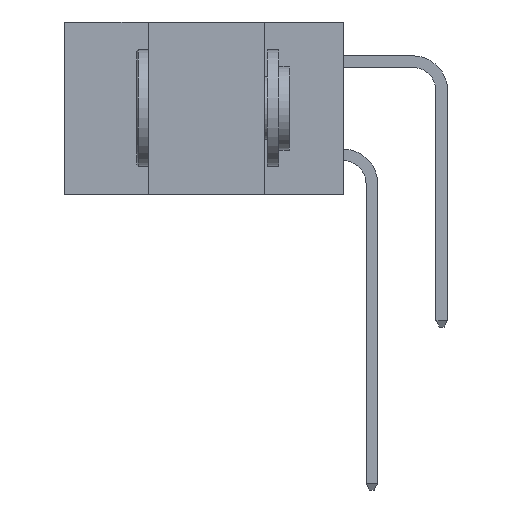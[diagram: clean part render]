
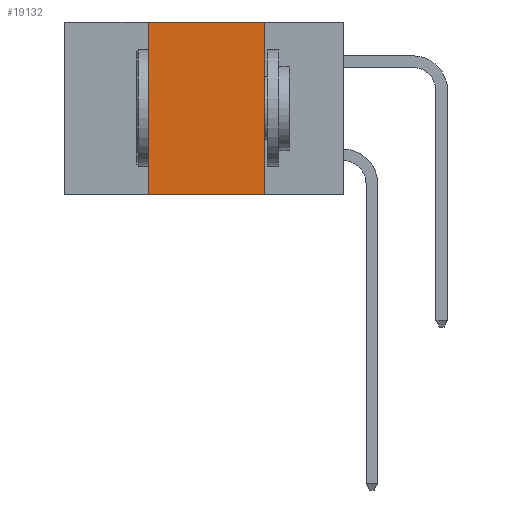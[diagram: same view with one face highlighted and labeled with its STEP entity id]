
A CAD part, left-side view. The second image highlights one B-rep face of the part: STEP entity #19132.
In plain terms, the highlighted planar face has unit normal (-1, 0, 0).
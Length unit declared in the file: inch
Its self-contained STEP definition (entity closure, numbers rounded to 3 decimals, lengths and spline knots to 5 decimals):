
#700 = CARTESIAN_POINT ( 'NONE',  ( 0., 0.6, 0. ) ) ;
#1573 = LINE ( 'NONE', #16615, #20217 ) ;
#2602 = DIRECTION ( 'NONE',  ( 1., 0., 0. ) ) ;
#3029 = ORIENTED_EDGE ( 'NONE', *, *, #15381, .T. ) ;
#3266 = VERTEX_POINT ( 'NONE', #19414 ) ;
#3692 = DIRECTION ( 'NONE',  ( 0., -1., 0. ) ) ;
#5593 = ORIENTED_EDGE ( 'NONE', *, *, #17843, .F. ) ;
#5947 = DIRECTION ( 'NONE',  ( 0., 0., -1. ) ) ;
#6161 = ORIENTED_EDGE ( 'NONE', *, *, #16584, .F. ) ;
#6325 = CARTESIAN_POINT ( 'NONE',  ( 0., 0.6, -0.37 ) ) ;
#7026 = FACE_OUTER_BOUND ( 'NONE', #20776, .T. ) ;
#7768 = DIRECTION ( 'NONE',  ( 0., 0., 1. ) ) ;
#7866 = VERTEX_POINT ( 'NONE', #9496 ) ;
#8141 = DIRECTION ( 'NONE',  ( 0., -1., 0. ) ) ;
#8465 = LINE ( 'NONE', #6325, #17462 ) ;
#8709 = VECTOR ( 'NONE', #5947, 39.37008 ) ;
#9181 = VECTOR ( 'NONE', #3692, 39.37008 ) ;
#9196 = VERTEX_POINT ( 'NONE', #13192 ) ;
#9496 = CARTESIAN_POINT ( 'NONE',  ( 0., 0.42, -0.37 ) ) ;
#10321 = AXIS2_PLACEMENT_3D ( 'NONE', #700, #2602, #15175 ) ;
#11581 = PLANE ( 'NONE',  #10321 ) ;
#13192 = CARTESIAN_POINT ( 'NONE',  ( 0., 0.17, 0. ) ) ;
#13944 = LINE ( 'NONE', #21557, #9181 ) ;
#15175 = DIRECTION ( 'NONE',  ( 0., 0., -1. ) ) ;
#15381 = EDGE_CURVE ( 'NONE', #7866, #3266, #8465, .T. ) ;
#16584 = EDGE_CURVE ( 'NONE', #7866, #19836, #1573, .T. ) ;
#16615 = CARTESIAN_POINT ( 'NONE',  ( 0., 0.42, -0.37 ) ) ;
#16671 = CARTESIAN_POINT ( 'NONE',  ( 0., 0.17, -0.37 ) ) ;
#16973 = CARTESIAN_POINT ( 'NONE',  ( 0., 0.42, 0. ) ) ;
#17462 = VECTOR ( 'NONE', #8141, 39.37008 ) ;
#17843 = EDGE_CURVE ( 'NONE', #19836, #9196, #13944, .T. ) ;
#19027 = EDGE_CURVE ( 'NONE', #9196, #3266, #23056, .T. ) ;
#19132 = ADVANCED_FACE ( 'NONE', ( #7026 ), #11581, .F. ) ;
#19380 = ORIENTED_EDGE ( 'NONE', *, *, #19027, .F. ) ;
#19414 = CARTESIAN_POINT ( 'NONE',  ( 0., 0.17, -0.37 ) ) ;
#19836 = VERTEX_POINT ( 'NONE', #16973 ) ;
#20217 = VECTOR ( 'NONE', #7768, 39.37008 ) ;
#20776 = EDGE_LOOP ( 'NONE', ( #19380, #5593, #6161, #3029 ) ) ;
#21557 = CARTESIAN_POINT ( 'NONE',  ( 0., 0.6, 0. ) ) ;
#23056 = LINE ( 'NONE', #16671, #8709 ) ;
